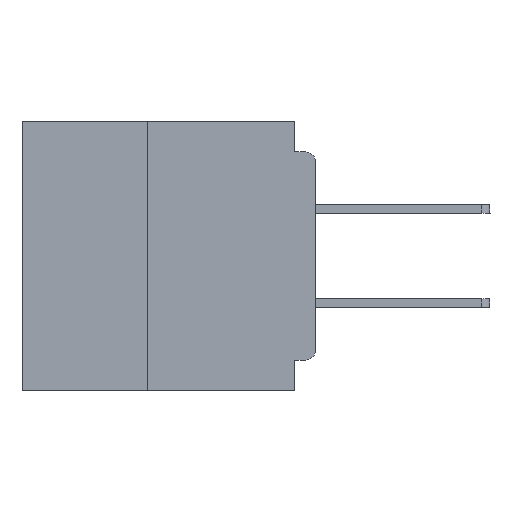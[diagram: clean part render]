
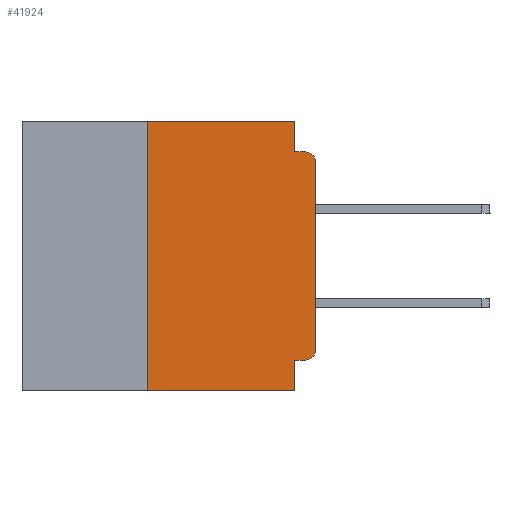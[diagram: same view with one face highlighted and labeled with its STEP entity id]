
A CAD part, left-side view. The second image highlights one B-rep face of the part: STEP entity #41924.
In plain terms, the highlighted planar face has unit normal (-1, 0, 0).
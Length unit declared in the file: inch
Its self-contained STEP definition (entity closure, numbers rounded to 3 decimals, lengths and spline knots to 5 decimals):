
#1703 = DIRECTION ( 'NONE',  ( 0., 0., -1. ) ) ;
#2617 = VERTEX_POINT ( 'NONE', #41861 ) ;
#3386 = LINE ( 'NONE', #6662, #44734 ) ;
#3456 = LINE ( 'NONE', #57417, #56848 ) ;
#4502 = AXIS2_PLACEMENT_3D ( 'NONE', #63621, #32973, #1703 ) ;
#5136 = DIRECTION ( 'NONE',  ( 0., 0., -1. ) ) ;
#6114 = EDGE_CURVE ( 'NONE', #51282, #18041, #43723, .T. ) ;
#6662 = CARTESIAN_POINT ( 'NONE',  ( 0., 0., 0. ) ) ;
#6663 = LINE ( 'NONE', #46372, #22545 ) ;
#8079 = EDGE_CURVE ( 'NONE', #17043, #11824, #31578, .T. ) ;
#8384 = VERTEX_POINT ( 'NONE', #9852 ) ;
#8843 = ORIENTED_EDGE ( 'NONE', *, *, #12734, .F. ) ;
#8899 = VERTEX_POINT ( 'NONE', #44806 ) ;
#9330 = EDGE_LOOP ( 'NONE', ( #51117, #32043, #30271, #52247, #51608, #8843, #44397, #14908, #38332, #33333 ) ) ;
#9852 = CARTESIAN_POINT ( 'NONE',  ( 0., 0.031, 0. ) ) ;
#11232 = EDGE_CURVE ( 'NONE', #8384, #53369, #6663, .T. ) ;
#11824 = VERTEX_POINT ( 'NONE', #25715 ) ;
#12733 = CARTESIAN_POINT ( 'NONE',  ( 0., 0., -0.355 ) ) ;
#12734 = EDGE_CURVE ( 'NONE', #17043, #54086, #64118, .T. ) ;
#13034 = VERTEX_POINT ( 'NONE', #37199 ) ;
#14449 = EDGE_CURVE ( 'NONE', #8899, #2617, #54338, .T. ) ;
#14908 = ORIENTED_EDGE ( 'NONE', *, *, #20160, .F. ) ;
#17043 = VERTEX_POINT ( 'NONE', #65306 ) ;
#17992 = DIRECTION ( 'NONE',  ( 0., 1., 0. ) ) ;
#18041 = VERTEX_POINT ( 'NONE', #49066 ) ;
#18291 = FACE_OUTER_BOUND ( 'NONE', #9330, .T. ) ;
#18445 = VECTOR ( 'NONE', #30383, 39.37008 ) ;
#19371 = CARTESIAN_POINT ( 'NONE',  ( 0., 0.25, -0.4 ) ) ;
#20085 = LINE ( 'NONE', #61039, #18445 ) ;
#20160 = EDGE_CURVE ( 'NONE', #13034, #11824, #3456, .T. ) ;
#22397 = DIRECTION ( 'NONE',  ( 1., 0., 0. ) ) ;
#22545 = VECTOR ( 'NONE', #5136, 39.37008 ) ;
#23209 = VECTOR ( 'NONE', #55310, 39.37008 ) ;
#23420 = DIRECTION ( 'NONE',  ( 0., -1., 0. ) ) ;
#25270 = CARTESIAN_POINT ( 'NONE',  ( 0., 0.031, -0.045 ) ) ;
#25715 = CARTESIAN_POINT ( 'NONE',  ( 0., 0.031, -0.4 ) ) ;
#27459 = CARTESIAN_POINT ( 'NONE',  ( 0., 0.015, -0.06 ) ) ;
#27961 = DIRECTION ( 'NONE',  ( 0., -1., 0. ) ) ;
#29310 = EDGE_CURVE ( 'NONE', #53369, #18041, #39339, .T. ) ;
#30271 = ORIENTED_EDGE ( 'NONE', *, *, #29310, .F. ) ;
#30383 = DIRECTION ( 'NONE',  ( 0., -1., 0. ) ) ;
#31578 = LINE ( 'NONE', #54107, #45164 ) ;
#32043 = ORIENTED_EDGE ( 'NONE', *, *, #6114, .T. ) ;
#32616 = DIRECTION ( 'NONE',  ( 0., 0., -1. ) ) ;
#32973 = DIRECTION ( 'NONE',  ( -1., 0., 0. ) ) ;
#33333 = ORIENTED_EDGE ( 'NONE', *, *, #14449, .T. ) ;
#35624 = EDGE_CURVE ( 'NONE', #54086, #8384, #20085, .T. ) ;
#37199 = CARTESIAN_POINT ( 'NONE',  ( 0., 0.031, -0.355 ) ) ;
#37821 = DIRECTION ( 'NONE',  ( 0., 0., 1. ) ) ;
#38332 = ORIENTED_EDGE ( 'NONE', *, *, #41397, .F. ) ;
#39339 = LINE ( 'NONE', #58570, #66568 ) ;
#40162 = VECTOR ( 'NONE', #17992, 39.37008 ) ;
#41397 = EDGE_CURVE ( 'NONE', #8899, #13034, #41744, .T. ) ;
#41744 = LINE ( 'NONE', #12733, #40162 ) ;
#41861 = CARTESIAN_POINT ( 'NONE',  ( 0., 0., -0.34 ) ) ;
#41924 = ADVANCED_FACE ( 'NONE', ( #18291 ), #47983, .F. ) ;
#41997 = DIRECTION ( 'NONE',  ( 0., 0., -1. ) ) ;
#43047 = EDGE_CURVE ( 'NONE', #2617, #51282, #3386, .T. ) ;
#43723 = CIRCLE ( 'NONE', #61282, 0.015 ) ;
#44397 = ORIENTED_EDGE ( 'NONE', *, *, #8079, .T. ) ;
#44734 = VECTOR ( 'NONE', #37821, 39.37008 ) ;
#44806 = CARTESIAN_POINT ( 'NONE',  ( 0., 0.015, -0.355 ) ) ;
#45164 = VECTOR ( 'NONE', #23420, 39.37008 ) ;
#46372 = CARTESIAN_POINT ( 'NONE',  ( 0., 0.031, 0. ) ) ;
#47983 = PLANE ( 'NONE',  #66924 ) ;
#48344 = CARTESIAN_POINT ( 'NONE',  ( 0., 0.25, 0. ) ) ;
#49066 = CARTESIAN_POINT ( 'NONE',  ( 0., 0.015, -0.045 ) ) ;
#51117 = ORIENTED_EDGE ( 'NONE', *, *, #43047, .T. ) ;
#51282 = VERTEX_POINT ( 'NONE', #59534 ) ;
#51608 = ORIENTED_EDGE ( 'NONE', *, *, #35624, .F. ) ;
#52247 = ORIENTED_EDGE ( 'NONE', *, *, #11232, .F. ) ;
#53128 = CARTESIAN_POINT ( 'NONE',  ( 0., 0.437, 0. ) ) ;
#53369 = VERTEX_POINT ( 'NONE', #25270 ) ;
#54086 = VERTEX_POINT ( 'NONE', #48344 ) ;
#54107 = CARTESIAN_POINT ( 'NONE',  ( 0., 0.437, -0.4 ) ) ;
#54338 = CIRCLE ( 'NONE', #4502, 0.015 ) ;
#55310 = DIRECTION ( 'NONE',  ( 0., 0., 1. ) ) ;
#56848 = VECTOR ( 'NONE', #41997, 39.37008 ) ;
#57417 = CARTESIAN_POINT ( 'NONE',  ( 0., 0.031, -0.4 ) ) ;
#58233 = DIRECTION ( 'NONE',  ( 0., 0., -1. ) ) ;
#58570 = CARTESIAN_POINT ( 'NONE',  ( 0., 0., -0.045 ) ) ;
#59534 = CARTESIAN_POINT ( 'NONE',  ( 0., 0., -0.06 ) ) ;
#61039 = CARTESIAN_POINT ( 'NONE',  ( 0., 0.437, 0. ) ) ;
#61282 = AXIS2_PLACEMENT_3D ( 'NONE', #27459, #63277, #32616 ) ;
#63277 = DIRECTION ( 'NONE',  ( -1., 0., 0. ) ) ;
#63621 = CARTESIAN_POINT ( 'NONE',  ( 0., 0.015, -0.34 ) ) ;
#64118 = LINE ( 'NONE', #19371, #23209 ) ;
#65306 = CARTESIAN_POINT ( 'NONE',  ( 0., 0.25, -0.4 ) ) ;
#66568 = VECTOR ( 'NONE', #27961, 39.37008 ) ;
#66924 = AXIS2_PLACEMENT_3D ( 'NONE', #53128, #22397, #58233 ) ;
